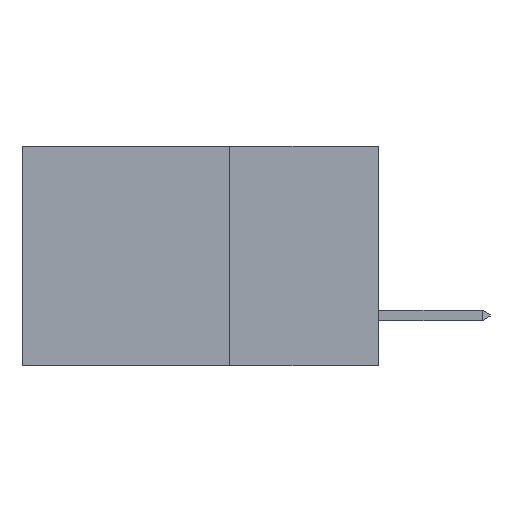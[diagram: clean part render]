
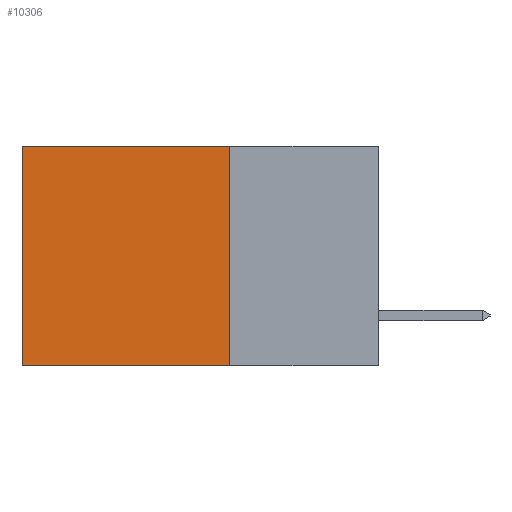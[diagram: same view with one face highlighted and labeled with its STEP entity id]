
A CAD part, left-side view. The second image highlights one B-rep face of the part: STEP entity #10306.
In plain terms, the highlighted planar face has unit normal (-1, 0, 0).
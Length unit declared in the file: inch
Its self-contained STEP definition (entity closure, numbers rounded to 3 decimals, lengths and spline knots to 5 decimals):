
#629 = EDGE_CURVE ( 'NONE', #10117, #19160, #18172, .T. ) ;
#1526 = CARTESIAN_POINT ( 'NONE',  ( 0.298, 0.25, 0. ) ) ;
#2233 = ORIENTED_EDGE ( 'NONE', *, *, #6048, .F. ) ;
#2385 = LINE ( 'NONE', #19109, #17945 ) ;
#2905 = VECTOR ( 'NONE', #19038, 39.37008 ) ;
#3192 = CARTESIAN_POINT ( 'NONE',  ( 0.298, 0.25, 0. ) ) ;
#4465 = EDGE_CURVE ( 'NONE', #17406, #21264, #12312, .T. ) ;
#5258 = CARTESIAN_POINT ( 'NONE',  ( 0.298, 0.25, -0.37 ) ) ;
#5753 = PLANE ( 'NONE',  #24266 ) ;
#6048 = EDGE_CURVE ( 'NONE', #17406, #10117, #2385, .T. ) ;
#6898 = ORIENTED_EDGE ( 'NONE', *, *, #629, .F. ) ;
#7556 = LINE ( 'NONE', #13248, #2905 ) ;
#7672 = CARTESIAN_POINT ( 'NONE',  ( 0.298, 0.25, 0. ) ) ;
#7763 = DIRECTION ( 'NONE',  ( 0., 0., -1. ) ) ;
#8493 = EDGE_CURVE ( 'NONE', #21264, #19160, #7556, .T. ) ;
#8727 = CARTESIAN_POINT ( 'NONE',  ( 0.298, 0.6, 0. ) ) ;
#9789 = EDGE_LOOP ( 'NONE', ( #21089, #6898, #2233, #12724 ) ) ;
#10117 = VERTEX_POINT ( 'NONE', #5258 ) ;
#10306 = ADVANCED_FACE ( 'NONE', ( #10846 ), #5753, .F. ) ;
#10846 = FACE_OUTER_BOUND ( 'NONE', #9789, .T. ) ;
#12312 = LINE ( 'NONE', #3192, #21875 ) ;
#12724 = ORIENTED_EDGE ( 'NONE', *, *, #4465, .T. ) ;
#13078 = VECTOR ( 'NONE', #15300, 39.37008 ) ;
#13248 = CARTESIAN_POINT ( 'NONE',  ( 0.298, 0.6, 0. ) ) ;
#14920 = DIRECTION ( 'NONE',  ( 0., 1., 0. ) ) ;
#15188 = CARTESIAN_POINT ( 'NONE',  ( 0.298, 0.25, -0.37 ) ) ;
#15300 = DIRECTION ( 'NONE',  ( 0., 1., 0. ) ) ;
#17406 = VERTEX_POINT ( 'NONE', #1526 ) ;
#17945 = VECTOR ( 'NONE', #24809, 39.37008 ) ;
#18172 = LINE ( 'NONE', #15188, #13078 ) ;
#19038 = DIRECTION ( 'NONE',  ( 0., 0., -1. ) ) ;
#19109 = CARTESIAN_POINT ( 'NONE',  ( 0.298, 0.25, 0. ) ) ;
#19160 = VERTEX_POINT ( 'NONE', #24341 ) ;
#19328 = DIRECTION ( 'NONE',  ( 1., 0., 0. ) ) ;
#21089 = ORIENTED_EDGE ( 'NONE', *, *, #8493, .T. ) ;
#21264 = VERTEX_POINT ( 'NONE', #8727 ) ;
#21875 = VECTOR ( 'NONE', #14920, 39.37008 ) ;
#24266 = AXIS2_PLACEMENT_3D ( 'NONE', #7672, #19328, #7763 ) ;
#24341 = CARTESIAN_POINT ( 'NONE',  ( 0.298, 0.6, -0.37 ) ) ;
#24809 = DIRECTION ( 'NONE',  ( 0., 0., -1. ) ) ;
